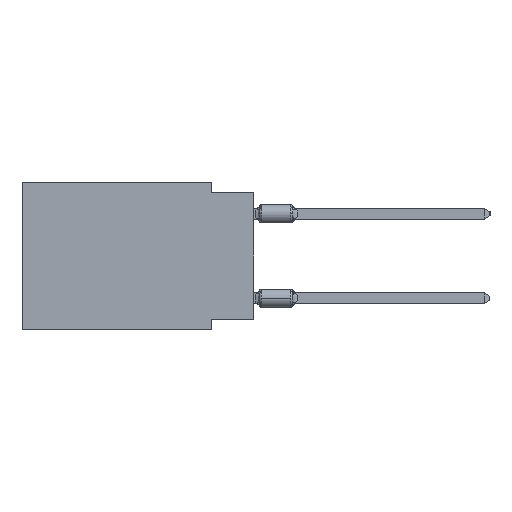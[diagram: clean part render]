
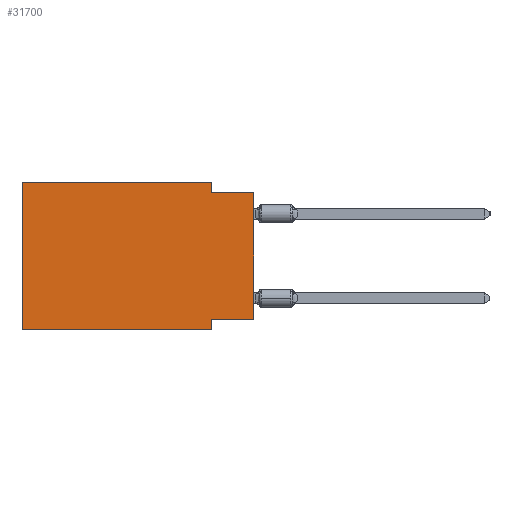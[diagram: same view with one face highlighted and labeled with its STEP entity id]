
A CAD part, left-side view. The second image highlights one B-rep face of the part: STEP entity #31700.
In plain terms, the highlighted planar face has unit normal (-1, 0, 0).
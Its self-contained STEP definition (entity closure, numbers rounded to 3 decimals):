
#118 = AXIS2_PLACEMENT_3D ( 'NONE', #8123, #28770, #16620 ) ;
#262 = CARTESIAN_POINT ( 'NONE',  ( 0., 2.54, -8.89 ) ) ;
#1151 = CARTESIAN_POINT ( 'NONE',  ( 0., 2.54, -0.635 ) ) ;
#1778 = LINE ( 'NONE', #19368, #15670 ) ;
#2553 = DIRECTION ( 'NONE',  ( 0., -1., 0. ) ) ;
#3453 = ORIENTED_EDGE ( 'NONE', *, *, #20903, .F. ) ;
#4203 = VECTOR ( 'NONE', #22155, 1000. ) ;
#4946 = LINE ( 'NONE', #33715, #25961 ) ;
#5111 = ORIENTED_EDGE ( 'NONE', *, *, #16212, .F. ) ;
#6053 = EDGE_CURVE ( 'NONE', #16523, #25826, #1778, .T. ) ;
#6085 = LINE ( 'NONE', #262, #10940 ) ;
#7083 = EDGE_CURVE ( 'NONE', #32705, #16434, #20033, .T. ) ;
#8123 = CARTESIAN_POINT ( 'NONE',  ( 0., 13.97, 0. ) ) ;
#10475 = EDGE_CURVE ( 'NONE', #32705, #35757, #24841, .T. ) ;
#10696 = ORIENTED_EDGE ( 'NONE', *, *, #6053, .F. ) ;
#10940 = VECTOR ( 'NONE', #12057, 1000. ) ;
#11070 = LINE ( 'NONE', #17229, #17685 ) ;
#11388 = EDGE_LOOP ( 'NONE', ( #26219, #3453, #5111, #36312, #10696, #34094, #32837, #26195 ) ) ;
#11649 = EDGE_CURVE ( 'NONE', #35757, #32761, #6085, .T. ) ;
#11664 = CARTESIAN_POINT ( 'NONE',  ( 0., 2.54, 0. ) ) ;
#12057 = DIRECTION ( 'NONE',  ( 0., 0., -1. ) ) ;
#12370 = CARTESIAN_POINT ( 'NONE',  ( 0., 0., -0.635 ) ) ;
#13528 = PLANE ( 'NONE',  #118 ) ;
#14097 = FACE_OUTER_BOUND ( 'NONE', #11388, .T. ) ;
#15133 = CARTESIAN_POINT ( 'NONE',  ( 0., 0., -8.255 ) ) ;
#15670 = VECTOR ( 'NONE', #37518, 1000. ) ;
#16212 = EDGE_CURVE ( 'NONE', #36662, #16399, #32265, .T. ) ;
#16399 = VERTEX_POINT ( 'NONE', #1151 ) ;
#16434 = VERTEX_POINT ( 'NONE', #12370 ) ;
#16523 = VERTEX_POINT ( 'NONE', #31472 ) ;
#16620 = DIRECTION ( 'NONE',  ( 0., 0., -1. ) ) ;
#16976 = VECTOR ( 'NONE', #17492, 1000. ) ;
#17229 = CARTESIAN_POINT ( 'NONE',  ( 0., 0., -0.635 ) ) ;
#17492 = DIRECTION ( 'NONE',  ( 0., 0., 1. ) ) ;
#17685 = VECTOR ( 'NONE', #2553, 1000. ) ;
#17856 = CARTESIAN_POINT ( 'NONE',  ( 0., 2.54, -8.89 ) ) ;
#19368 = CARTESIAN_POINT ( 'NONE',  ( 0., 13.97, 0. ) ) ;
#19679 = CARTESIAN_POINT ( 'NONE',  ( 0., 13.97, -8.89 ) ) ;
#20033 = LINE ( 'NONE', #20580, #16976 ) ;
#20580 = CARTESIAN_POINT ( 'NONE',  ( 0., 0., 0. ) ) ;
#20903 = EDGE_CURVE ( 'NONE', #16399, #16434, #11070, .T. ) ;
#22155 = DIRECTION ( 'NONE',  ( 0., 1., 0. ) ) ;
#23566 = CARTESIAN_POINT ( 'NONE',  ( 0., 2.54, 0. ) ) ;
#24841 = LINE ( 'NONE', #28125, #4203 ) ;
#25125 = EDGE_CURVE ( 'NONE', #25826, #36662, #4946, .T. ) ;
#25446 = VECTOR ( 'NONE', #29741, 1000. ) ;
#25642 = DIRECTION ( 'NONE',  ( 0., -1., 0. ) ) ;
#25826 = VERTEX_POINT ( 'NONE', #28022 ) ;
#25961 = VECTOR ( 'NONE', #30809, 1000. ) ;
#26195 = ORIENTED_EDGE ( 'NONE', *, *, #10475, .F. ) ;
#26219 = ORIENTED_EDGE ( 'NONE', *, *, #7083, .T. ) ;
#26509 = EDGE_CURVE ( 'NONE', #16523, #32761, #37258, .T. ) ;
#28022 = CARTESIAN_POINT ( 'NONE',  ( 0., 13.97, 0. ) ) ;
#28125 = CARTESIAN_POINT ( 'NONE',  ( 0., 0., -8.255 ) ) ;
#28770 = DIRECTION ( 'NONE',  ( 1., 0., 0. ) ) ;
#29122 = VECTOR ( 'NONE', #25642, 1000. ) ;
#29741 = DIRECTION ( 'NONE',  ( 0., 0., -1. ) ) ;
#30809 = DIRECTION ( 'NONE',  ( 0., -1., 0. ) ) ;
#31472 = CARTESIAN_POINT ( 'NONE',  ( 0., 13.97, -8.89 ) ) ;
#31700 = ADVANCED_FACE ( 'NONE', ( #14097 ), #13528, .F. ) ;
#32265 = LINE ( 'NONE', #23566, #25446 ) ;
#32705 = VERTEX_POINT ( 'NONE', #15133 ) ;
#32761 = VERTEX_POINT ( 'NONE', #17856 ) ;
#32837 = ORIENTED_EDGE ( 'NONE', *, *, #11649, .F. ) ;
#33715 = CARTESIAN_POINT ( 'NONE',  ( 0., 13.97, 0. ) ) ;
#34094 = ORIENTED_EDGE ( 'NONE', *, *, #26509, .T. ) ;
#35757 = VERTEX_POINT ( 'NONE', #37147 ) ;
#36312 = ORIENTED_EDGE ( 'NONE', *, *, #25125, .F. ) ;
#36662 = VERTEX_POINT ( 'NONE', #11664 ) ;
#37147 = CARTESIAN_POINT ( 'NONE',  ( 0., 2.54, -8.255 ) ) ;
#37258 = LINE ( 'NONE', #19679, #29122 ) ;
#37518 = DIRECTION ( 'NONE',  ( 0., 0., 1. ) ) ;
